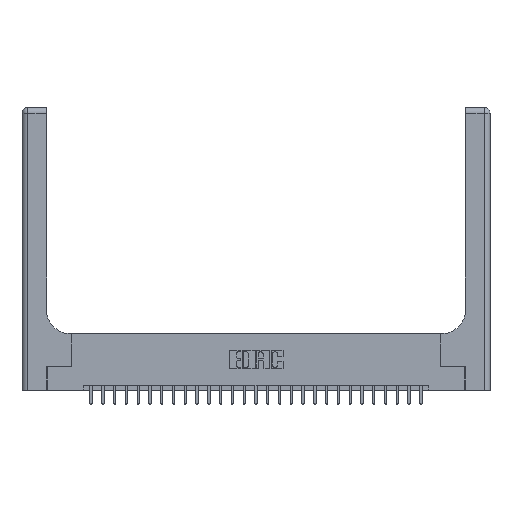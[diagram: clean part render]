
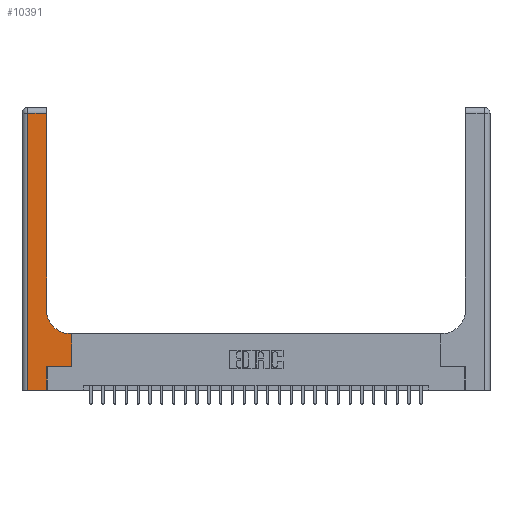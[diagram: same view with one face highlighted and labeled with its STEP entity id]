
A CAD part, top view. The second image highlights one B-rep face of the part: STEP entity #10391.
In plain terms, the highlighted planar face has unit normal (0, 0, 1).
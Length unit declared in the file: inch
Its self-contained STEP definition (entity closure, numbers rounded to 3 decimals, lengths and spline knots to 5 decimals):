
#62 = VERTEX_POINT ( 'NONE', #19707 ) ;
#236 = CARTESIAN_POINT ( 'NONE',  ( 0.06, 2.94, 0.37 ) ) ;
#1161 = PLANE ( 'NONE',  #13861 ) ;
#1759 = DIRECTION ( 'NONE',  ( 0., 0., -1. ) ) ;
#2173 = EDGE_CURVE ( 'NONE', #22268, #62, #10075, .T. ) ;
#3502 = DIRECTION ( 'NONE',  ( 0., 1., 0. ) ) ;
#3625 = LINE ( 'NONE', #20352, #7504 ) ;
#4032 = VECTOR ( 'NONE', #14711, 39.37008 ) ;
#4983 = VERTEX_POINT ( 'NONE', #8255 ) ;
#5026 = VERTEX_POINT ( 'NONE', #23195 ) ;
#5028 = CARTESIAN_POINT ( 'NONE',  ( 0., 3., 0.37 ) ) ;
#5773 = EDGE_CURVE ( 'NONE', #4983, #6979, #7214, .T. ) ;
#5813 = FACE_OUTER_BOUND ( 'NONE', #23046, .T. ) ;
#6147 = CARTESIAN_POINT ( 'NONE',  ( 0.26, 3., 0.37 ) ) ;
#6398 = EDGE_CURVE ( 'NONE', #6979, #18982, #3625, .T. ) ;
#6572 = CARTESIAN_POINT ( 'NONE',  ( 0.265, 0., 0.37 ) ) ;
#6647 = VECTOR ( 'NONE', #10889, 39.37008 ) ;
#6949 = DIRECTION ( 'NONE',  ( 1., 0., 0. ) ) ;
#6979 = VERTEX_POINT ( 'NONE', #23295 ) ;
#7214 = LINE ( 'NONE', #15365, #11781 ) ;
#7387 = VERTEX_POINT ( 'NONE', #8259 ) ;
#7454 = ORIENTED_EDGE ( 'NONE', *, *, #11508, .T. ) ;
#7504 = VECTOR ( 'NONE', #19872, 39.37008 ) ;
#7814 = LINE ( 'NONE', #19860, #13822 ) ;
#7932 = EDGE_CURVE ( 'NONE', #62, #4983, #24818, .T. ) ;
#8255 = CARTESIAN_POINT ( 'NONE',  ( 0.265, 0.25, 0.37 ) ) ;
#8259 = CARTESIAN_POINT ( 'NONE',  ( 0.51, 0.6, 0.37 ) ) ;
#8305 = LINE ( 'NONE', #16982, #6647 ) ;
#8409 = ORIENTED_EDGE ( 'NONE', *, *, #20435, .T. ) ;
#9789 = DIRECTION ( 'NONE',  ( -1., 0., 0. ) ) ;
#9898 = CARTESIAN_POINT ( 'NONE',  ( 0.06, 0., 0.37 ) ) ;
#10075 = LINE ( 'NONE', #22565, #26294 ) ;
#10391 = ADVANCED_FACE ( 'NONE', ( #5813 ), #1161, .F. ) ;
#10476 = DIRECTION ( 'NONE',  ( 1., 0., 0. ) ) ;
#10741 = ORIENTED_EDGE ( 'NONE', *, *, #15704, .T. ) ;
#10889 = DIRECTION ( 'NONE',  ( -1., 0., 0. ) ) ;
#11465 = VERTEX_POINT ( 'NONE', #20314 ) ;
#11508 = EDGE_CURVE ( 'NONE', #5026, #11922, #8305, .T. ) ;
#11781 = VECTOR ( 'NONE', #6949, 39.37008 ) ;
#11919 = CARTESIAN_POINT ( 'NONE',  ( 0.06, 3., 0.37 ) ) ;
#11922 = VERTEX_POINT ( 'NONE', #236 ) ;
#12121 = DIRECTION ( 'NONE',  ( 1., 0., 0. ) ) ;
#12158 = LINE ( 'NONE', #6147, #24329 ) ;
#12756 = ORIENTED_EDGE ( 'NONE', *, *, #7932, .T. ) ;
#13812 = LINE ( 'NONE', #11919, #25632 ) ;
#13822 = VECTOR ( 'NONE', #15981, 39.37008 ) ;
#13861 = AXIS2_PLACEMENT_3D ( 'NONE', #5028, #1759, #9789 ) ;
#14711 = DIRECTION ( 'NONE',  ( 0., 1., 0. ) ) ;
#15365 = CARTESIAN_POINT ( 'NONE',  ( 0.265, 0.25, 0.37 ) ) ;
#15704 = EDGE_CURVE ( 'NONE', #11465, #5026, #12158, .T. ) ;
#15981 = DIRECTION ( 'NONE',  ( -1., 0., 0. ) ) ;
#16982 = CARTESIAN_POINT ( 'NONE',  ( 0., 2.94, 0.37 ) ) ;
#18982 = VERTEX_POINT ( 'NONE', #19895 ) ;
#19393 = ORIENTED_EDGE ( 'NONE', *, *, #25025, .T. ) ;
#19707 = CARTESIAN_POINT ( 'NONE',  ( 0.265, 0., 0.37 ) ) ;
#19860 = CARTESIAN_POINT ( 'NONE',  ( 0.26, 0.6, 0.37 ) ) ;
#19872 = DIRECTION ( 'NONE',  ( 0., 1., 0. ) ) ;
#19895 = CARTESIAN_POINT ( 'NONE',  ( 0.528, 0.6, 0.37 ) ) ;
#20314 = CARTESIAN_POINT ( 'NONE',  ( 0.26, 0.85, 0.37 ) ) ;
#20352 = CARTESIAN_POINT ( 'NONE',  ( 0.528, 0.25, 0.37 ) ) ;
#20435 = EDGE_CURVE ( 'NONE', #7387, #11465, #21809, .T. ) ;
#20549 = EDGE_CURVE ( 'NONE', #11922, #22268, #13812, .T. ) ;
#21369 = AXIS2_PLACEMENT_3D ( 'NONE', #25743, #22497, #12121 ) ;
#21798 = ORIENTED_EDGE ( 'NONE', *, *, #6398, .T. ) ;
#21809 = CIRCLE ( 'NONE', #21369, 0.25 ) ;
#21823 = ORIENTED_EDGE ( 'NONE', *, *, #2173, .T. ) ;
#22268 = VERTEX_POINT ( 'NONE', #9898 ) ;
#22497 = DIRECTION ( 'NONE',  ( 0., 0., -1. ) ) ;
#22565 = CARTESIAN_POINT ( 'NONE',  ( 0., 0., 0.37 ) ) ;
#23046 = EDGE_LOOP ( 'NONE', ( #10741, #7454, #26041, #21823, #12756, #25605, #21798, #19393, #8409 ) ) ;
#23195 = CARTESIAN_POINT ( 'NONE',  ( 0.26, 2.94, 0.37 ) ) ;
#23295 = CARTESIAN_POINT ( 'NONE',  ( 0.528, 0.25, 0.37 ) ) ;
#24329 = VECTOR ( 'NONE', #3502, 39.37008 ) ;
#24818 = LINE ( 'NONE', #6572, #4032 ) ;
#25025 = EDGE_CURVE ( 'NONE', #18982, #7387, #7814, .T. ) ;
#25605 = ORIENTED_EDGE ( 'NONE', *, *, #5773, .T. ) ;
#25632 = VECTOR ( 'NONE', #25916, 39.37008 ) ;
#25743 = CARTESIAN_POINT ( 'NONE',  ( 0.51, 0.85, 0.37 ) ) ;
#25916 = DIRECTION ( 'NONE',  ( 0., -1., 0. ) ) ;
#26041 = ORIENTED_EDGE ( 'NONE', *, *, #20549, .T. ) ;
#26294 = VECTOR ( 'NONE', #10476, 39.37008 ) ;
